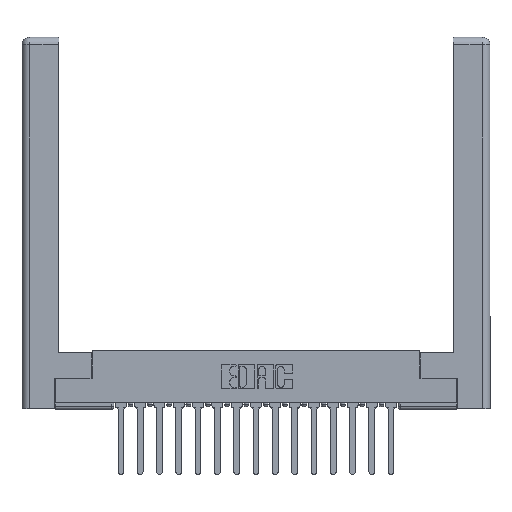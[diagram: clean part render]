
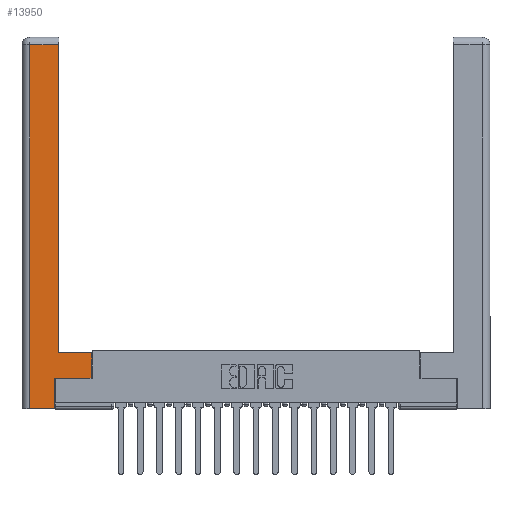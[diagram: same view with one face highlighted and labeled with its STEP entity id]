
A CAD part, top view. The second image highlights one B-rep face of the part: STEP entity #13950.
In plain terms, the highlighted planar face has unit normal (0, 0, 1).
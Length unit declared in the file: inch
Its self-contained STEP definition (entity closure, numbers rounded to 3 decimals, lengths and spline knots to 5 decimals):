
#113 = ORIENTED_EDGE ( 'NONE', *, *, #9790, .T. ) ;
#125 = LINE ( 'NONE', #8362, #15946 ) ;
#352 = VERTEX_POINT ( 'NONE', #16202 ) ;
#546 = CARTESIAN_POINT ( 'NONE',  ( 0.265, 0.245, 0. ) ) ;
#1070 = EDGE_CURVE ( 'NONE', #11193, #2133, #10986, .T. ) ;
#1220 = VECTOR ( 'NONE', #6217, 39.37008 ) ;
#1265 = CARTESIAN_POINT ( 'NONE',  ( 0.295, 2.94, 0. ) ) ;
#1682 = PLANE ( 'NONE',  #10944 ) ;
#1768 = DIRECTION ( 'NONE',  ( -1., 0., 0. ) ) ;
#2133 = VERTEX_POINT ( 'NONE', #7933 ) ;
#2489 = ORIENTED_EDGE ( 'NONE', *, *, #15420, .T. ) ;
#2652 = VERTEX_POINT ( 'NONE', #5362 ) ;
#2942 = CARTESIAN_POINT ( 'NONE',  ( 0.0615, 0., 0. ) ) ;
#2943 = VECTOR ( 'NONE', #15573, 39.37008 ) ;
#3668 = CARTESIAN_POINT ( 'NONE',  ( 0.0615, 2.94, 0. ) ) ;
#4650 = ORIENTED_EDGE ( 'NONE', *, *, #18094, .T. ) ;
#4950 = VECTOR ( 'NONE', #18666, 39.37008 ) ;
#5362 = CARTESIAN_POINT ( 'NONE',  ( 0.265, 0.245, 0. ) ) ;
#6111 = CARTESIAN_POINT ( 'NONE',  ( 0.295, 0.45, 0. ) ) ;
#6217 = DIRECTION ( 'NONE',  ( 1., 0., 0. ) ) ;
#6901 = EDGE_LOOP ( 'NONE', ( #4650, #10182, #15384, #10565, #2489, #16275, #11926, #113 ) ) ;
#7552 = EDGE_CURVE ( 'NONE', #2652, #10390, #14009, .T. ) ;
#7933 = CARTESIAN_POINT ( 'NONE',  ( 0.0615, 2.94, 0. ) ) ;
#8190 = DIRECTION ( 'NONE',  ( 0., 1., 0. ) ) ;
#8202 = LINE ( 'NONE', #14073, #4950 ) ;
#8362 = CARTESIAN_POINT ( 'NONE',  ( 0.295, 3., 0. ) ) ;
#9273 = EDGE_CURVE ( 'NONE', #2133, #14289, #12522, .T. ) ;
#9790 = EDGE_CURVE ( 'NONE', #15522, #11667, #8202, .T. ) ;
#9904 = VECTOR ( 'NONE', #16547, 39.37008 ) ;
#9912 = CARTESIAN_POINT ( 'NONE',  ( 0.565, 0.45, 0. ) ) ;
#9936 = VECTOR ( 'NONE', #18420, 39.37008 ) ;
#10182 = ORIENTED_EDGE ( 'NONE', *, *, #1070, .T. ) ;
#10390 = VERTEX_POINT ( 'NONE', #13238 ) ;
#10565 = ORIENTED_EDGE ( 'NONE', *, *, #18656, .T. ) ;
#10588 = CARTESIAN_POINT ( 'NONE',  ( 0.0615, 0., 0. ) ) ;
#10829 = FACE_OUTER_BOUND ( 'NONE', #6901, .T. ) ;
#10944 = AXIS2_PLACEMENT_3D ( 'NONE', #11927, #13858, #1768 ) ;
#10986 = LINE ( 'NONE', #3668, #2943 ) ;
#11193 = VERTEX_POINT ( 'NONE', #1265 ) ;
#11461 = LINE ( 'NONE', #18697, #11873 ) ;
#11667 = VERTEX_POINT ( 'NONE', #6111 ) ;
#11873 = VECTOR ( 'NONE', #12933, 39.37008 ) ;
#11926 = ORIENTED_EDGE ( 'NONE', *, *, #14098, .T. ) ;
#11927 = CARTESIAN_POINT ( 'NONE',  ( 0., 0., 0. ) ) ;
#12522 = LINE ( 'NONE', #10588, #9904 ) ;
#12933 = DIRECTION ( 'NONE',  ( 1., 0., 0. ) ) ;
#13238 = CARTESIAN_POINT ( 'NONE',  ( 0.565, 0.245, 0. ) ) ;
#13858 = DIRECTION ( 'NONE',  ( 0., 0., -1. ) ) ;
#13950 = ADVANCED_FACE ( 'NONE', ( #10829 ), #1682, .F. ) ;
#14009 = LINE ( 'NONE', #18035, #1220 ) ;
#14073 = CARTESIAN_POINT ( 'NONE',  ( 0.295, 0.45, 0. ) ) ;
#14098 = EDGE_CURVE ( 'NONE', #10390, #15522, #14246, .T. ) ;
#14246 = LINE ( 'NONE', #16887, #15939 ) ;
#14289 = VERTEX_POINT ( 'NONE', #2942 ) ;
#15193 = LINE ( 'NONE', #546, #9936 ) ;
#15384 = ORIENTED_EDGE ( 'NONE', *, *, #9273, .T. ) ;
#15420 = EDGE_CURVE ( 'NONE', #352, #2652, #15193, .T. ) ;
#15522 = VERTEX_POINT ( 'NONE', #9912 ) ;
#15573 = DIRECTION ( 'NONE',  ( -1., 0., 0. ) ) ;
#15939 = VECTOR ( 'NONE', #8190, 39.37008 ) ;
#15946 = VECTOR ( 'NONE', #17554, 39.37008 ) ;
#16202 = CARTESIAN_POINT ( 'NONE',  ( 0.265, 0., 0. ) ) ;
#16275 = ORIENTED_EDGE ( 'NONE', *, *, #7552, .T. ) ;
#16547 = DIRECTION ( 'NONE',  ( 0., -1., 0. ) ) ;
#16887 = CARTESIAN_POINT ( 'NONE',  ( 0.565, 0.45, 0. ) ) ;
#17554 = DIRECTION ( 'NONE',  ( 0., 1., 0. ) ) ;
#18035 = CARTESIAN_POINT ( 'NONE',  ( 0.565, 0.245, 0. ) ) ;
#18094 = EDGE_CURVE ( 'NONE', #11667, #11193, #125, .T. ) ;
#18420 = DIRECTION ( 'NONE',  ( 0., 1., 0. ) ) ;
#18656 = EDGE_CURVE ( 'NONE', #14289, #352, #11461, .T. ) ;
#18666 = DIRECTION ( 'NONE',  ( -1., 0., 0. ) ) ;
#18697 = CARTESIAN_POINT ( 'NONE',  ( 0.265, 0., 0. ) ) ;
